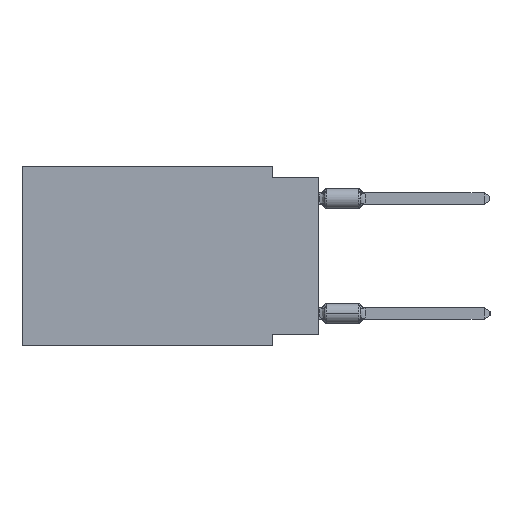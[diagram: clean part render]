
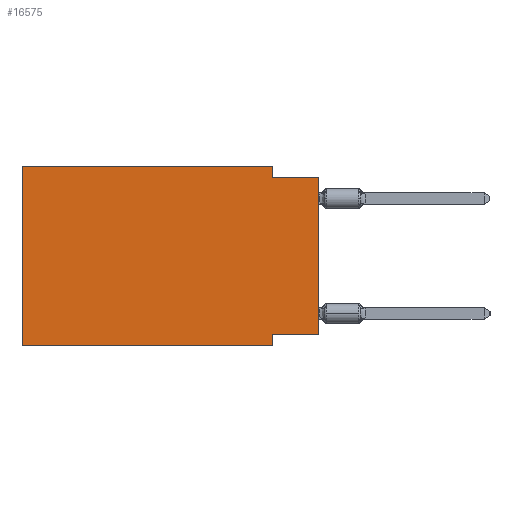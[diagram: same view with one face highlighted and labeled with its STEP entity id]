
A CAD part, left-side view. The second image highlights one B-rep face of the part: STEP entity #16575.
In plain terms, the highlighted planar face has unit normal (-1, 0, 0).
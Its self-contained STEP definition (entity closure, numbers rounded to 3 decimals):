
#1140 = ORIENTED_EDGE ( 'NONE', *, *, #9071, .F. ) ;
#1319 = PLANE ( 'NONE',  #30116 ) ;
#1371 = LINE ( 'NONE', #25330, #8196 ) ;
#1414 = VERTEX_POINT ( 'NONE', #3174 ) ;
#1596 = LINE ( 'NONE', #11212, #4309 ) ;
#2048 = VERTEX_POINT ( 'NONE', #4075 ) ;
#3174 = CARTESIAN_POINT ( 'NONE',  ( 0., 0., -9.271 ) ) ;
#3382 = FACE_OUTER_BOUND ( 'NONE', #4090, .T. ) ;
#3938 = CARTESIAN_POINT ( 'NONE',  ( 0., 0., -9.271 ) ) ;
#4061 = DIRECTION ( 'NONE',  ( 0., -1., 0. ) ) ;
#4075 = CARTESIAN_POINT ( 'NONE',  ( 0., 2.54, -0.635 ) ) ;
#4090 = EDGE_LOOP ( 'NONE', ( #16224, #31074, #26041, #13333, #1140, #12542, #5813, #13448 ) ) ;
#4121 = LINE ( 'NONE', #4434, #25593 ) ;
#4309 = VECTOR ( 'NONE', #16244, 1000. ) ;
#4404 = EDGE_CURVE ( 'NONE', #2048, #27213, #1371, .T. ) ;
#4434 = CARTESIAN_POINT ( 'NONE',  ( 0., 16.383, 0. ) ) ;
#5224 = CARTESIAN_POINT ( 'NONE',  ( 0., 2.54, 0. ) ) ;
#5380 = LINE ( 'NONE', #5224, #13501 ) ;
#5663 = EDGE_CURVE ( 'NONE', #1414, #10717, #15297, .T. ) ;
#5813 = ORIENTED_EDGE ( 'NONE', *, *, #13574, .F. ) ;
#5911 = DIRECTION ( 'NONE',  ( 0., 0., -1. ) ) ;
#5977 = VERTEX_POINT ( 'NONE', #12589 ) ;
#8196 = VECTOR ( 'NONE', #4061, 1000. ) ;
#8522 = DIRECTION ( 'NONE',  ( 0., 1., 0. ) ) ;
#9071 = EDGE_CURVE ( 'NONE', #5977, #10914, #22727, .T. ) ;
#9598 = CARTESIAN_POINT ( 'NONE',  ( 0., 2.54, 0. ) ) ;
#10717 = VERTEX_POINT ( 'NONE', #20646 ) ;
#10914 = VERTEX_POINT ( 'NONE', #12750 ) ;
#11212 = CARTESIAN_POINT ( 'NONE',  ( 0., 16.383, -9.906 ) ) ;
#11404 = DIRECTION ( 'NONE',  ( 0., 0., -1. ) ) ;
#11736 = LINE ( 'NONE', #26245, #19503 ) ;
#11887 = EDGE_CURVE ( 'NONE', #5977, #16582, #1596, .T. ) ;
#12542 = ORIENTED_EDGE ( 'NONE', *, *, #11887, .T. ) ;
#12589 = CARTESIAN_POINT ( 'NONE',  ( 0., 16.383, -9.906 ) ) ;
#12750 = CARTESIAN_POINT ( 'NONE',  ( 0., 16.383, 0. ) ) ;
#12764 = VERTEX_POINT ( 'NONE', #9598 ) ;
#13143 = CARTESIAN_POINT ( 'NONE',  ( 0., 2.54, -9.906 ) ) ;
#13333 = ORIENTED_EDGE ( 'NONE', *, *, #28362, .F. ) ;
#13448 = ORIENTED_EDGE ( 'NONE', *, *, #5663, .F. ) ;
#13501 = VECTOR ( 'NONE', #31091, 1000. ) ;
#13574 = EDGE_CURVE ( 'NONE', #10717, #16582, #23845, .T. ) ;
#15297 = LINE ( 'NONE', #3938, #23346 ) ;
#15977 = DIRECTION ( 'NONE',  ( 0., 0., 1. ) ) ;
#16224 = ORIENTED_EDGE ( 'NONE', *, *, #27106, .T. ) ;
#16244 = DIRECTION ( 'NONE',  ( 0., -1., 0. ) ) ;
#16575 = ADVANCED_FACE ( 'NONE', ( #3382 ), #1319, .F. ) ;
#16582 = VERTEX_POINT ( 'NONE', #13143 ) ;
#19503 = VECTOR ( 'NONE', #15977, 1000. ) ;
#20072 = DIRECTION ( 'NONE',  ( 1., 0., 0. ) ) ;
#20646 = CARTESIAN_POINT ( 'NONE',  ( 0., 2.54, -9.271 ) ) ;
#20971 = DIRECTION ( 'NONE',  ( 0., -1., 0. ) ) ;
#22289 = CARTESIAN_POINT ( 'NONE',  ( 0., 16.383, 0. ) ) ;
#22306 = VECTOR ( 'NONE', #25413, 1000. ) ;
#22727 = LINE ( 'NONE', #27794, #22306 ) ;
#23346 = VECTOR ( 'NONE', #8522, 1000. ) ;
#23845 = LINE ( 'NONE', #28759, #27967 ) ;
#24483 = CARTESIAN_POINT ( 'NONE',  ( 0., 0., -0.635 ) ) ;
#25330 = CARTESIAN_POINT ( 'NONE',  ( 0., 0., -0.635 ) ) ;
#25413 = DIRECTION ( 'NONE',  ( 0., 0., 1. ) ) ;
#25593 = VECTOR ( 'NONE', #20971, 1000. ) ;
#26041 = ORIENTED_EDGE ( 'NONE', *, *, #28480, .F. ) ;
#26245 = CARTESIAN_POINT ( 'NONE',  ( 0., 0., 0. ) ) ;
#27106 = EDGE_CURVE ( 'NONE', #1414, #27213, #11736, .T. ) ;
#27213 = VERTEX_POINT ( 'NONE', #24483 ) ;
#27794 = CARTESIAN_POINT ( 'NONE',  ( 0., 16.383, 0. ) ) ;
#27967 = VECTOR ( 'NONE', #11404, 1000. ) ;
#28362 = EDGE_CURVE ( 'NONE', #10914, #12764, #4121, .T. ) ;
#28480 = EDGE_CURVE ( 'NONE', #12764, #2048, #5380, .T. ) ;
#28759 = CARTESIAN_POINT ( 'NONE',  ( 0., 2.54, -9.906 ) ) ;
#30116 = AXIS2_PLACEMENT_3D ( 'NONE', #22289, #20072, #5911 ) ;
#31074 = ORIENTED_EDGE ( 'NONE', *, *, #4404, .F. ) ;
#31091 = DIRECTION ( 'NONE',  ( 0., 0., -1. ) ) ;
